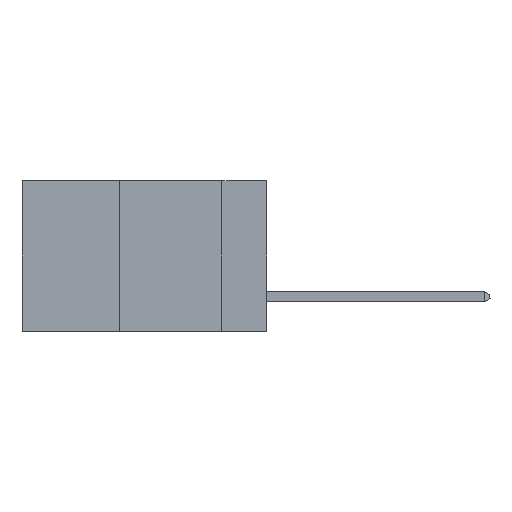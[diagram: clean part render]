
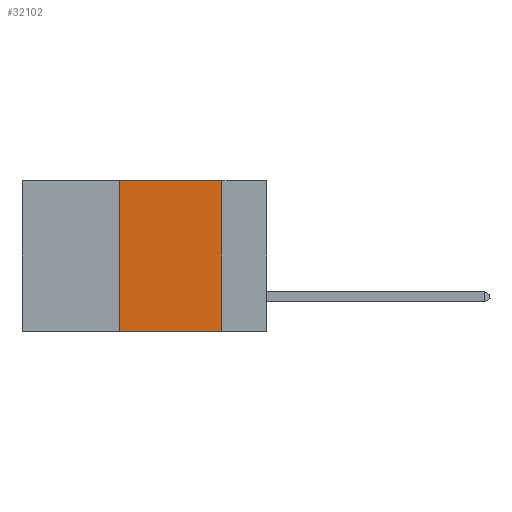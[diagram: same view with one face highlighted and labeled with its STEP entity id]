
A CAD part, left-side view. The second image highlights one B-rep face of the part: STEP entity #32102.
In plain terms, the highlighted planar face has unit normal (-1, 0, 0).
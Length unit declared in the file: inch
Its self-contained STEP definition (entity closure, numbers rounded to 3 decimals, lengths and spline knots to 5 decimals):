
#681 = VECTOR ( 'NONE', #7699, 39.37008 ) ;
#846 = ORIENTED_EDGE ( 'NONE', *, *, #26769, .F. ) ;
#1466 = CARTESIAN_POINT ( 'NONE',  ( 0., 0.6, -0.37 ) ) ;
#3019 = EDGE_CURVE ( 'NONE', #14490, #5250, #30412, .T. ) ;
#3661 = VERTEX_POINT ( 'NONE', #7842 ) ;
#4837 = EDGE_LOOP ( 'NONE', ( #17268, #846, #7150, #18604 ) ) ;
#5250 = VERTEX_POINT ( 'NONE', #16295 ) ;
#7150 = ORIENTED_EDGE ( 'NONE', *, *, #3019, .F. ) ;
#7482 = LINE ( 'NONE', #20175, #681 ) ;
#7699 = DIRECTION ( 'NONE',  ( 0., -1., 0. ) ) ;
#7836 = CARTESIAN_POINT ( 'NONE',  ( 0., 0.36, 0. ) ) ;
#7842 = CARTESIAN_POINT ( 'NONE',  ( 0., 0.11, -0.37 ) ) ;
#10089 = EDGE_CURVE ( 'NONE', #14490, #3661, #32006, .T. ) ;
#11447 = DIRECTION ( 'NONE',  ( 1., 0., 0. ) ) ;
#12496 = FACE_OUTER_BOUND ( 'NONE', #4837, .T. ) ;
#12904 = VERTEX_POINT ( 'NONE', #17148 ) ;
#14079 = DIRECTION ( 'NONE',  ( 0., 0., -1. ) ) ;
#14399 = DIRECTION ( 'NONE',  ( 0., -1., 0. ) ) ;
#14490 = VERTEX_POINT ( 'NONE', #28361 ) ;
#16295 = CARTESIAN_POINT ( 'NONE',  ( 0., 0.36, 0. ) ) ;
#17148 = CARTESIAN_POINT ( 'NONE',  ( 0., 0.11, 0. ) ) ;
#17268 = ORIENTED_EDGE ( 'NONE', *, *, #29829, .F. ) ;
#18604 = ORIENTED_EDGE ( 'NONE', *, *, #10089, .T. ) ;
#18903 = CARTESIAN_POINT ( 'NONE',  ( 0., 0.6, 0. ) ) ;
#20175 = CARTESIAN_POINT ( 'NONE',  ( 0., 0.6, 0. ) ) ;
#21058 = VECTOR ( 'NONE', #14079, 39.37008 ) ;
#21870 = CARTESIAN_POINT ( 'NONE',  ( 0., 0.11, 0. ) ) ;
#25677 = DIRECTION ( 'NONE',  ( 0., 0., 1. ) ) ;
#26085 = AXIS2_PLACEMENT_3D ( 'NONE', #18903, #11447, #31631 ) ;
#26769 = EDGE_CURVE ( 'NONE', #5250, #12904, #7482, .T. ) ;
#27314 = VECTOR ( 'NONE', #14399, 39.37008 ) ;
#27836 = LINE ( 'NONE', #21870, #21058 ) ;
#28361 = CARTESIAN_POINT ( 'NONE',  ( 0., 0.36, -0.37 ) ) ;
#29829 = EDGE_CURVE ( 'NONE', #12904, #3661, #27836, .T. ) ;
#30412 = LINE ( 'NONE', #7836, #32415 ) ;
#31402 = PLANE ( 'NONE',  #26085 ) ;
#31631 = DIRECTION ( 'NONE',  ( 0., 0., -1. ) ) ;
#32006 = LINE ( 'NONE', #1466, #27314 ) ;
#32102 = ADVANCED_FACE ( 'NONE', ( #12496 ), #31402, .F. ) ;
#32415 = VECTOR ( 'NONE', #25677, 39.37008 ) ;
